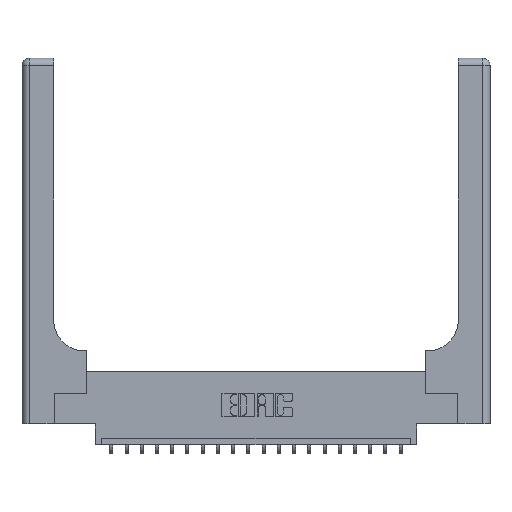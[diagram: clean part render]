
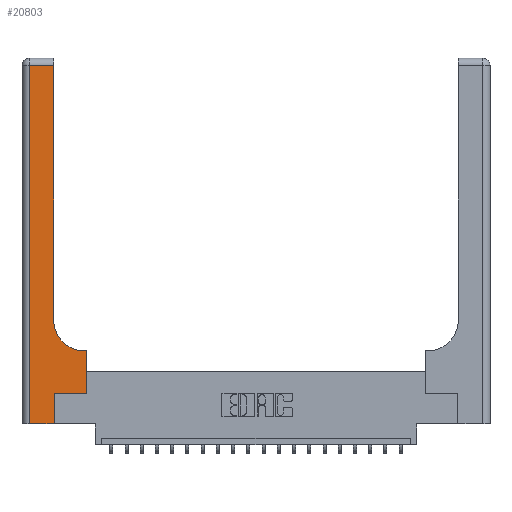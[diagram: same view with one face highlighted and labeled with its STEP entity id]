
A CAD part, top view. The second image highlights one B-rep face of the part: STEP entity #20803.
In plain terms, the highlighted planar face has unit normal (0, 0, 1).
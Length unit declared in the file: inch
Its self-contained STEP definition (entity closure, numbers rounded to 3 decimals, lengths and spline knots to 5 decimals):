
#711 = CARTESIAN_POINT ( 'NONE',  ( 0., 2.94, 0.37 ) ) ;
#788 = AXIS2_PLACEMENT_3D ( 'NONE', #17580, #7918, #15968 ) ;
#907 = ORIENTED_EDGE ( 'NONE', *, *, #10954, .T. ) ;
#952 = VERTEX_POINT ( 'NONE', #4506 ) ;
#1485 = LINE ( 'NONE', #19296, #17751 ) ;
#1716 = DIRECTION ( 'NONE',  ( 0., 1., 0. ) ) ;
#2094 = ORIENTED_EDGE ( 'NONE', *, *, #14085, .T. ) ;
#2891 = CARTESIAN_POINT ( 'NONE',  ( 0.06, 3., 0.37 ) ) ;
#2977 = VECTOR ( 'NONE', #20944, 39.37008 ) ;
#3054 = EDGE_CURVE ( 'NONE', #18474, #11941, #6461, .T. ) ;
#3435 = CARTESIAN_POINT ( 'NONE',  ( 0.528, 0.25, 0.37 ) ) ;
#4135 = EDGE_CURVE ( 'NONE', #5851, #19810, #8649, .T. ) ;
#4500 = LINE ( 'NONE', #2891, #5501 ) ;
#4506 = CARTESIAN_POINT ( 'NONE',  ( 0.265, 0.25, 0.37 ) ) ;
#4611 = DIRECTION ( 'NONE',  ( -1., 0., 0. ) ) ;
#5047 = EDGE_CURVE ( 'NONE', #13069, #7814, #1485, .T. ) ;
#5501 = VECTOR ( 'NONE', #18012, 39.37008 ) ;
#5697 = VERTEX_POINT ( 'NONE', #20434 ) ;
#5851 = VERTEX_POINT ( 'NONE', #18930 ) ;
#6461 = LINE ( 'NONE', #7649, #2977 ) ;
#6653 = ORIENTED_EDGE ( 'NONE', *, *, #10674, .T. ) ;
#6905 = CIRCLE ( 'NONE', #18554, 0.25 ) ;
#7449 = EDGE_CURVE ( 'NONE', #19810, #18474, #4500, .T. ) ;
#7453 = VECTOR ( 'NONE', #20022, 39.37008 ) ;
#7649 = CARTESIAN_POINT ( 'NONE',  ( 0., 0., 0.37 ) ) ;
#7814 = VERTEX_POINT ( 'NONE', #20466 ) ;
#7918 = DIRECTION ( 'NONE',  ( 0., 0., -1. ) ) ;
#7995 = VECTOR ( 'NONE', #20121, 39.37008 ) ;
#8649 = LINE ( 'NONE', #711, #7453 ) ;
#8762 = CARTESIAN_POINT ( 'NONE',  ( 0.06, 2.94, 0.37 ) ) ;
#9442 = CARTESIAN_POINT ( 'NONE',  ( 0.528, 0.25, 0.37 ) ) ;
#9720 = CARTESIAN_POINT ( 'NONE',  ( 0.528, 0.6, 0.37 ) ) ;
#10541 = CARTESIAN_POINT ( 'NONE',  ( 0.265, 0., 0.37 ) ) ;
#10674 = EDGE_CURVE ( 'NONE', #7814, #5697, #6905, .T. ) ;
#10785 = CARTESIAN_POINT ( 'NONE',  ( 0.265, 0., 0.37 ) ) ;
#10954 = EDGE_CURVE ( 'NONE', #19248, #13069, #20911, .T. ) ;
#11153 = DIRECTION ( 'NONE',  ( 0., 1., 0. ) ) ;
#11480 = CARTESIAN_POINT ( 'NONE',  ( 0.26, 3., 0.37 ) ) ;
#11941 = VERTEX_POINT ( 'NONE', #10541 ) ;
#12539 = CARTESIAN_POINT ( 'NONE',  ( 0.265, 0.25, 0.37 ) ) ;
#12632 = DIRECTION ( 'NONE',  ( 1., 0., 0. ) ) ;
#13069 = VERTEX_POINT ( 'NONE', #9720 ) ;
#13079 = LINE ( 'NONE', #11480, #18310 ) ;
#13904 = LINE ( 'NONE', #10785, #7995 ) ;
#13970 = ORIENTED_EDGE ( 'NONE', *, *, #19466, .T. ) ;
#13983 = EDGE_CURVE ( 'NONE', #5697, #5851, #13079, .T. ) ;
#14085 = EDGE_CURVE ( 'NONE', #11941, #952, #13904, .T. ) ;
#14557 = CARTESIAN_POINT ( 'NONE',  ( 0.06, 0., 0.37 ) ) ;
#14594 = ORIENTED_EDGE ( 'NONE', *, *, #5047, .T. ) ;
#15075 = ORIENTED_EDGE ( 'NONE', *, *, #13983, .T. ) ;
#15141 = VECTOR ( 'NONE', #11153, 39.37008 ) ;
#15681 = EDGE_LOOP ( 'NONE', ( #15075, #19868, #16965, #15693, #2094, #13970, #907, #14594, #6653 ) ) ;
#15693 = ORIENTED_EDGE ( 'NONE', *, *, #3054, .T. ) ;
#15968 = DIRECTION ( 'NONE',  ( -1., 0., 0. ) ) ;
#16965 = ORIENTED_EDGE ( 'NONE', *, *, #7449, .T. ) ;
#17574 = LINE ( 'NONE', #12539, #19253 ) ;
#17580 = CARTESIAN_POINT ( 'NONE',  ( 0., 3., 0.37 ) ) ;
#17751 = VECTOR ( 'NONE', #4611, 39.37008 ) ;
#17789 = PLANE ( 'NONE',  #788 ) ;
#18012 = DIRECTION ( 'NONE',  ( 0., -1., 0. ) ) ;
#18248 = CARTESIAN_POINT ( 'NONE',  ( 0.51, 0.85, 0.37 ) ) ;
#18310 = VECTOR ( 'NONE', #1716, 39.37008 ) ;
#18474 = VERTEX_POINT ( 'NONE', #14557 ) ;
#18554 = AXIS2_PLACEMENT_3D ( 'NONE', #18248, #19652, #20064 ) ;
#18930 = CARTESIAN_POINT ( 'NONE',  ( 0.26, 2.94, 0.37 ) ) ;
#19248 = VERTEX_POINT ( 'NONE', #3435 ) ;
#19253 = VECTOR ( 'NONE', #12632, 39.37008 ) ;
#19296 = CARTESIAN_POINT ( 'NONE',  ( 0.26, 0.6, 0.37 ) ) ;
#19466 = EDGE_CURVE ( 'NONE', #952, #19248, #17574, .T. ) ;
#19652 = DIRECTION ( 'NONE',  ( 0., 0., -1. ) ) ;
#19810 = VERTEX_POINT ( 'NONE', #8762 ) ;
#19868 = ORIENTED_EDGE ( 'NONE', *, *, #4135, .T. ) ;
#20022 = DIRECTION ( 'NONE',  ( -1., 0., 0. ) ) ;
#20064 = DIRECTION ( 'NONE',  ( 1., 0., 0. ) ) ;
#20121 = DIRECTION ( 'NONE',  ( 0., 1., 0. ) ) ;
#20434 = CARTESIAN_POINT ( 'NONE',  ( 0.26, 0.85, 0.37 ) ) ;
#20466 = CARTESIAN_POINT ( 'NONE',  ( 0.51, 0.6, 0.37 ) ) ;
#20803 = ADVANCED_FACE ( 'NONE', ( #21117 ), #17789, .F. ) ;
#20911 = LINE ( 'NONE', #9442, #15141 ) ;
#20944 = DIRECTION ( 'NONE',  ( 1., 0., 0. ) ) ;
#21117 = FACE_OUTER_BOUND ( 'NONE', #15681, .T. ) ;
